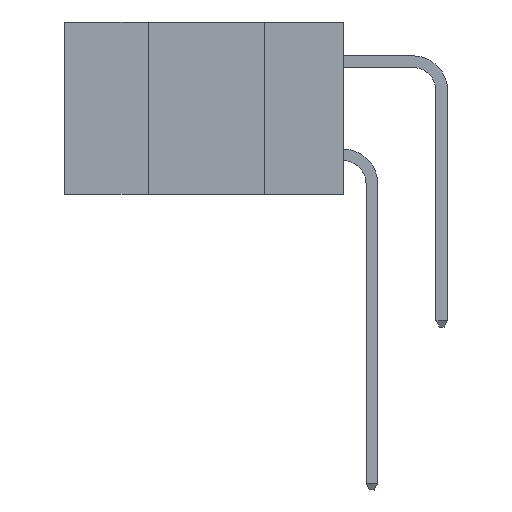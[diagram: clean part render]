
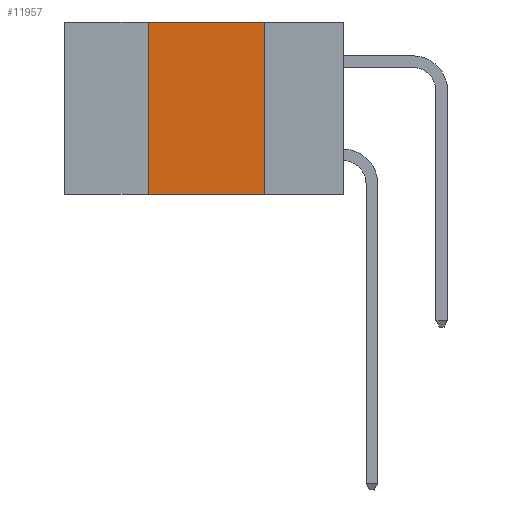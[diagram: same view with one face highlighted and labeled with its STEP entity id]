
A CAD part, left-side view. The second image highlights one B-rep face of the part: STEP entity #11957.
In plain terms, the highlighted planar face has unit normal (-1, 0, 0).
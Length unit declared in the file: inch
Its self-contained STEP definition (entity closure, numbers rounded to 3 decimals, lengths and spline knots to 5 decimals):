
#556 = EDGE_CURVE ( 'NONE', #6279, #27321, #26753, .T. ) ;
#707 = EDGE_CURVE ( 'NONE', #7358, #26893, #24463, .T. ) ;
#1166 = ORIENTED_EDGE ( 'NONE', *, *, #14069, .F. ) ;
#4756 = DIRECTION ( 'NONE',  ( 0., 0., -1. ) ) ;
#6279 = VERTEX_POINT ( 'NONE', #10880 ) ;
#6615 = CARTESIAN_POINT ( 'NONE',  ( 0., 0.6, 0. ) ) ;
#7272 = CARTESIAN_POINT ( 'NONE',  ( 0., 0.6, -0.37 ) ) ;
#7358 = VERTEX_POINT ( 'NONE', #21036 ) ;
#8067 = ORIENTED_EDGE ( 'NONE', *, *, #556, .F. ) ;
#8085 = LINE ( 'NONE', #14794, #22321 ) ;
#9013 = CARTESIAN_POINT ( 'NONE',  ( 0., 0.42, 0. ) ) ;
#9099 = DIRECTION ( 'NONE',  ( 1., 0., 0. ) ) ;
#9447 = AXIS2_PLACEMENT_3D ( 'NONE', #6615, #9099, #13864 ) ;
#10880 = CARTESIAN_POINT ( 'NONE',  ( 0., 0.42, 0. ) ) ;
#11050 = VECTOR ( 'NONE', #19213, 39.37008 ) ;
#11434 = VECTOR ( 'NONE', #26073, 39.37008 ) ;
#11672 = EDGE_LOOP ( 'NONE', ( #21839, #8067, #1166, #28234 ) ) ;
#11957 = ADVANCED_FACE ( 'NONE', ( #30803 ), #16534, .F. ) ;
#13864 = DIRECTION ( 'NONE',  ( 0., 0., -1. ) ) ;
#14069 = EDGE_CURVE ( 'NONE', #7358, #6279, #31798, .T. ) ;
#14794 = CARTESIAN_POINT ( 'NONE',  ( 0., 0.17, 0. ) ) ;
#16534 = PLANE ( 'NONE',  #9447 ) ;
#19213 = DIRECTION ( 'NONE',  ( 0., -1., 0. ) ) ;
#19735 = DIRECTION ( 'NONE',  ( 0., -1., 0. ) ) ;
#19902 = EDGE_CURVE ( 'NONE', #27321, #26893, #8085, .T. ) ;
#20212 = VECTOR ( 'NONE', #19735, 39.37008 ) ;
#20250 = CARTESIAN_POINT ( 'NONE',  ( 0., 0.17, 0. ) ) ;
#21036 = CARTESIAN_POINT ( 'NONE',  ( 0., 0.42, -0.37 ) ) ;
#21166 = CARTESIAN_POINT ( 'NONE',  ( 0., 0.17, -0.37 ) ) ;
#21839 = ORIENTED_EDGE ( 'NONE', *, *, #19902, .F. ) ;
#22321 = VECTOR ( 'NONE', #4756, 39.37008 ) ;
#24463 = LINE ( 'NONE', #7272, #20212 ) ;
#26073 = DIRECTION ( 'NONE',  ( 0., 0., 1. ) ) ;
#26753 = LINE ( 'NONE', #31465, #11050 ) ;
#26893 = VERTEX_POINT ( 'NONE', #21166 ) ;
#27321 = VERTEX_POINT ( 'NONE', #20250 ) ;
#28234 = ORIENTED_EDGE ( 'NONE', *, *, #707, .T. ) ;
#30803 = FACE_OUTER_BOUND ( 'NONE', #11672, .T. ) ;
#31465 = CARTESIAN_POINT ( 'NONE',  ( 0., 0.6, 0. ) ) ;
#31798 = LINE ( 'NONE', #9013, #11434 ) ;
